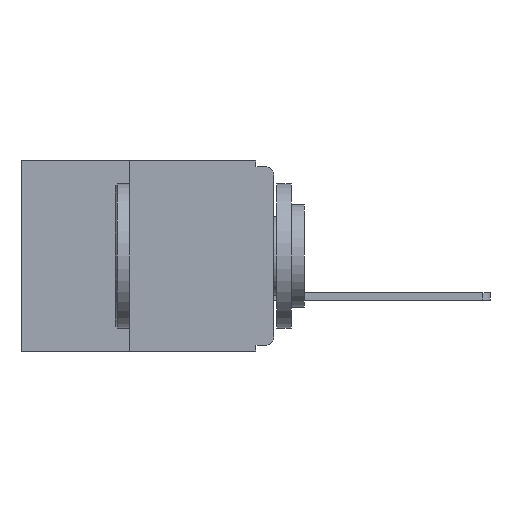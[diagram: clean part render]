
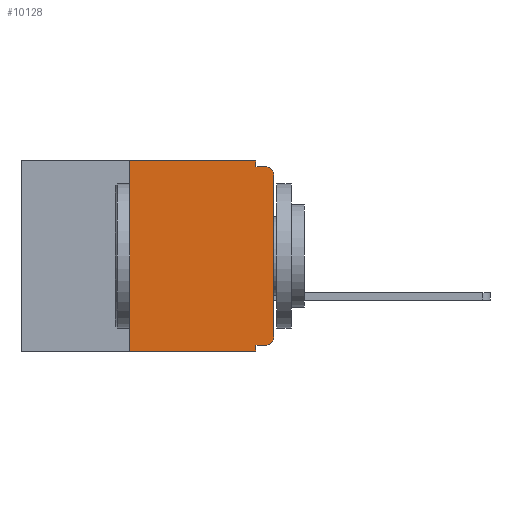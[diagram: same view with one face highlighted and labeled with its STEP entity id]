
A CAD part, left-side view. The second image highlights one B-rep face of the part: STEP entity #10128.
In plain terms, the highlighted planar face has unit normal (-1, 0, 0).
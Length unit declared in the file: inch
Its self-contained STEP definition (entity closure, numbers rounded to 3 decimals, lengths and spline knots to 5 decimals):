
#265 = DIRECTION ( 'NONE',  ( 0., 0., 1. ) ) ;
#337 = CARTESIAN_POINT ( 'NONE',  ( 0., 0.25, 0. ) ) ;
#666 = CARTESIAN_POINT ( 'NONE',  ( 0., 0.25, -0.33 ) ) ;
#892 = VECTOR ( 'NONE', #265, 39.37008 ) ;
#929 = FACE_OUTER_BOUND ( 'NONE', #8901, .T. ) ;
#1068 = LINE ( 'NONE', #666, #892 ) ;
#1733 = CARTESIAN_POINT ( 'NONE',  ( 0., 0., -0.32 ) ) ;
#2069 = VERTEX_POINT ( 'NONE', #16999 ) ;
#2241 = VERTEX_POINT ( 'NONE', #10584 ) ;
#2279 = ORIENTED_EDGE ( 'NONE', *, *, #3137, .T. ) ;
#2406 = VERTEX_POINT ( 'NONE', #14837 ) ;
#3046 = ORIENTED_EDGE ( 'NONE', *, *, #15389, .T. ) ;
#3137 = EDGE_CURVE ( 'NONE', #3962, #3144, #16243, .T. ) ;
#3144 = VERTEX_POINT ( 'NONE', #11900 ) ;
#3321 = AXIS2_PLACEMENT_3D ( 'NONE', #14339, #13736, #13630 ) ;
#3526 = CARTESIAN_POINT ( 'NONE',  ( 0., 0., 0. ) ) ;
#3746 = EDGE_CURVE ( 'NONE', #4115, #14057, #17178, .T. ) ;
#3782 = VECTOR ( 'NONE', #6892, 39.37008 ) ;
#3802 = LINE ( 'NONE', #1733, #3782 ) ;
#3962 = VERTEX_POINT ( 'NONE', #15808 ) ;
#4115 = VERTEX_POINT ( 'NONE', #7859 ) ;
#4166 = EDGE_CURVE ( 'NONE', #2241, #14057, #18154, .T. ) ;
#4224 = DIRECTION ( 'NONE',  ( 0., 0., -1. ) ) ;
#4482 = CARTESIAN_POINT ( 'NONE',  ( 0., 0.031, -0.33 ) ) ;
#5002 = DIRECTION ( 'NONE',  ( 0., 0., 1. ) ) ;
#5056 = DIRECTION ( 'NONE',  ( -1., 0., 0. ) ) ;
#5222 = CARTESIAN_POINT ( 'NONE',  ( 0., 0.015, -0.305 ) ) ;
#5434 = DIRECTION ( 'NONE',  ( 0., 0., -1. ) ) ;
#5566 = LINE ( 'NONE', #8162, #5588 ) ;
#5588 = VECTOR ( 'NONE', #8611, 39.37008 ) ;
#6146 = ORIENTED_EDGE ( 'NONE', *, *, #7837, .F. ) ;
#6754 = ORIENTED_EDGE ( 'NONE', *, *, #17331, .T. ) ;
#6892 = DIRECTION ( 'NONE',  ( 0., 1., 0. ) ) ;
#7104 = ORIENTED_EDGE ( 'NONE', *, *, #13404, .F. ) ;
#7371 = EDGE_CURVE ( 'NONE', #2069, #12445, #5566, .T. ) ;
#7525 = VECTOR ( 'NONE', #11088, 39.37008 ) ;
#7571 = LINE ( 'NONE', #11343, #7525 ) ;
#7728 = ORIENTED_EDGE ( 'NONE', *, *, #8716, .F. ) ;
#7837 = EDGE_CURVE ( 'NONE', #2406, #2241, #3802, .T. ) ;
#7859 = CARTESIAN_POINT ( 'NONE',  ( 0., 0.25, -0.33 ) ) ;
#8162 = CARTESIAN_POINT ( 'NONE',  ( 0., 0.031, 0. ) ) ;
#8611 = DIRECTION ( 'NONE',  ( 0., 0., -1. ) ) ;
#8716 = EDGE_CURVE ( 'NONE', #4115, #13653, #1068, .T. ) ;
#8901 = EDGE_LOOP ( 'NONE', ( #2279, #3046, #13143, #14227, #7104, #7728, #17012, #17739, #6146, #6754 ) ) ;
#9220 = VERTEX_POINT ( 'NONE', #10908 ) ;
#9235 = DIRECTION ( 'NONE',  ( 0., 0., -1. ) ) ;
#9238 = DIRECTION ( 'NONE',  ( -1., 0., 0. ) ) ;
#9263 = CARTESIAN_POINT ( 'NONE',  ( 0., 0.015, -0.025 ) ) ;
#9365 = CIRCLE ( 'NONE', #18697, 0.015 ) ;
#9728 = VECTOR ( 'NONE', #14769, 39.37008 ) ;
#9812 = LINE ( 'NONE', #14590, #9728 ) ;
#10128 = ADVANCED_FACE ( 'NONE', ( #929 ), #13777, .F. ) ;
#10584 = CARTESIAN_POINT ( 'NONE',  ( 0., 0.031, -0.32 ) ) ;
#10908 = CARTESIAN_POINT ( 'NONE',  ( 0., 0.015, -0.01 ) ) ;
#11088 = DIRECTION ( 'NONE',  ( 0., -1., 0. ) ) ;
#11343 = CARTESIAN_POINT ( 'NONE',  ( 0., 0.437, 0. ) ) ;
#11900 = CARTESIAN_POINT ( 'NONE',  ( 0., 0., -0.025 ) ) ;
#12304 = CARTESIAN_POINT ( 'NONE',  ( 0., 0.437, -0.33 ) ) ;
#12445 = VERTEX_POINT ( 'NONE', #13179 ) ;
#12465 = DIRECTION ( 'NONE',  ( 0., -1., 0. ) ) ;
#13143 = ORIENTED_EDGE ( 'NONE', *, *, #18322, .F. ) ;
#13179 = CARTESIAN_POINT ( 'NONE',  ( 0., 0.031, -0.01 ) ) ;
#13404 = EDGE_CURVE ( 'NONE', #13653, #2069, #7571, .T. ) ;
#13630 = DIRECTION ( 'NONE',  ( 0., 0., -1. ) ) ;
#13653 = VERTEX_POINT ( 'NONE', #337 ) ;
#13736 = DIRECTION ( 'NONE',  ( 1., 0., 0. ) ) ;
#13777 = PLANE ( 'NONE',  #3321 ) ;
#14057 = VERTEX_POINT ( 'NONE', #15295 ) ;
#14078 = AXIS2_PLACEMENT_3D ( 'NONE', #5222, #5056, #4224 ) ;
#14227 = ORIENTED_EDGE ( 'NONE', *, *, #7371, .F. ) ;
#14339 = CARTESIAN_POINT ( 'NONE',  ( 0., 0.437, 0. ) ) ;
#14590 = CARTESIAN_POINT ( 'NONE',  ( 0., 0., -0.01 ) ) ;
#14769 = DIRECTION ( 'NONE',  ( 0., -1., 0. ) ) ;
#14837 = CARTESIAN_POINT ( 'NONE',  ( 0., 0.015, -0.32 ) ) ;
#15295 = CARTESIAN_POINT ( 'NONE',  ( 0., 0.031, -0.33 ) ) ;
#15389 = EDGE_CURVE ( 'NONE', #3144, #9220, #9365, .T. ) ;
#15808 = CARTESIAN_POINT ( 'NONE',  ( 0., 0., -0.305 ) ) ;
#16071 = VECTOR ( 'NONE', #5002, 39.37008 ) ;
#16243 = LINE ( 'NONE', #3526, #16071 ) ;
#16999 = CARTESIAN_POINT ( 'NONE',  ( 0., 0.031, 0. ) ) ;
#17012 = ORIENTED_EDGE ( 'NONE', *, *, #3746, .T. ) ;
#17079 = VECTOR ( 'NONE', #12465, 39.37008 ) ;
#17178 = LINE ( 'NONE', #12304, #17079 ) ;
#17320 = CIRCLE ( 'NONE', #14078, 0.015 ) ;
#17331 = EDGE_CURVE ( 'NONE', #2406, #3962, #17320, .T. ) ;
#17739 = ORIENTED_EDGE ( 'NONE', *, *, #4166, .F. ) ;
#18154 = LINE ( 'NONE', #4482, #18348 ) ;
#18322 = EDGE_CURVE ( 'NONE', #12445, #9220, #9812, .T. ) ;
#18348 = VECTOR ( 'NONE', #5434, 39.37008 ) ;
#18697 = AXIS2_PLACEMENT_3D ( 'NONE', #9263, #9238, #9235 ) ;
